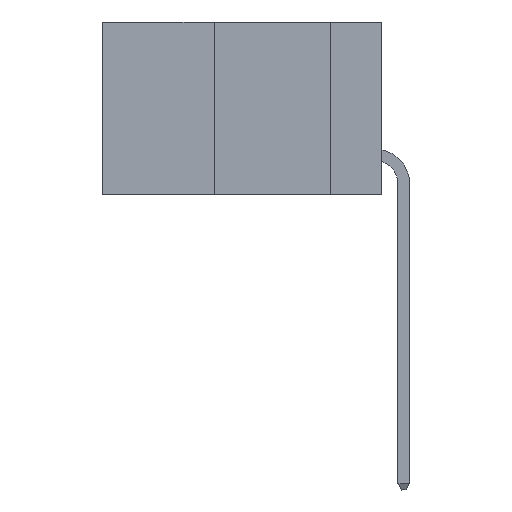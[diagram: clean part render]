
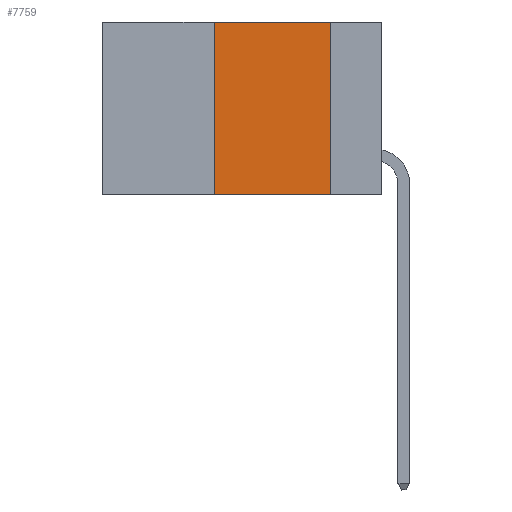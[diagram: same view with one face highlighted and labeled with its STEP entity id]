
A CAD part, left-side view. The second image highlights one B-rep face of the part: STEP entity #7759.
In plain terms, the highlighted planar face has unit normal (-1, 0, 0).
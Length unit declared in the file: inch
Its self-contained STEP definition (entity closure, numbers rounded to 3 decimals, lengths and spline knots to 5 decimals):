
#589 = EDGE_CURVE ( 'NONE', #13950, #16127, #8821, .T. ) ;
#635 = CARTESIAN_POINT ( 'NONE',  ( 0., 0.36, -0.37 ) ) ;
#652 = ORIENTED_EDGE ( 'NONE', *, *, #11546, .F. ) ;
#664 = CARTESIAN_POINT ( 'NONE',  ( 0., 0.6, -0.37 ) ) ;
#1356 = VECTOR ( 'NONE', #12120, 39.37008 ) ;
#2468 = VECTOR ( 'NONE', #7566, 39.37008 ) ;
#3319 = EDGE_CURVE ( 'NONE', #15656, #16127, #4731, .T. ) ;
#3501 = EDGE_LOOP ( 'NONE', ( #10491, #652, #5030, #10488 ) ) ;
#3700 = LINE ( 'NONE', #4114, #10033 ) ;
#3900 = CARTESIAN_POINT ( 'NONE',  ( 0., 0.6, 0. ) ) ;
#4114 = CARTESIAN_POINT ( 'NONE',  ( 0., 0.6, 0. ) ) ;
#4138 = CARTESIAN_POINT ( 'NONE',  ( 0., 0.36, 0. ) ) ;
#4293 = CARTESIAN_POINT ( 'NONE',  ( 0., 0.36, 0. ) ) ;
#4709 = VERTEX_POINT ( 'NONE', #4293 ) ;
#4731 = LINE ( 'NONE', #664, #1356 ) ;
#5030 = ORIENTED_EDGE ( 'NONE', *, *, #7220, .F. ) ;
#6456 = DIRECTION ( 'NONE',  ( 1., 0., 0. ) ) ;
#7220 = EDGE_CURVE ( 'NONE', #15656, #4709, #9380, .T. ) ;
#7566 = DIRECTION ( 'NONE',  ( 0., 0., -1. ) ) ;
#7759 = ADVANCED_FACE ( 'NONE', ( #15041 ), #11476, .F. ) ;
#8821 = LINE ( 'NONE', #15148, #2468 ) ;
#8979 = CARTESIAN_POINT ( 'NONE',  ( 0., 0.11, 0. ) ) ;
#8985 = DIRECTION ( 'NONE',  ( 0., 0., -1. ) ) ;
#9380 = LINE ( 'NONE', #4138, #12157 ) ;
#10033 = VECTOR ( 'NONE', #12933, 39.37008 ) ;
#10488 = ORIENTED_EDGE ( 'NONE', *, *, #3319, .T. ) ;
#10491 = ORIENTED_EDGE ( 'NONE', *, *, #589, .F. ) ;
#10588 = CARTESIAN_POINT ( 'NONE',  ( 0., 0.11, -0.37 ) ) ;
#11476 = PLANE ( 'NONE',  #13377 ) ;
#11546 = EDGE_CURVE ( 'NONE', #4709, #13950, #3700, .T. ) ;
#11601 = DIRECTION ( 'NONE',  ( 0., 0., 1. ) ) ;
#12120 = DIRECTION ( 'NONE',  ( 0., -1., 0. ) ) ;
#12157 = VECTOR ( 'NONE', #11601, 39.37008 ) ;
#12933 = DIRECTION ( 'NONE',  ( 0., -1., 0. ) ) ;
#13377 = AXIS2_PLACEMENT_3D ( 'NONE', #3900, #6456, #8985 ) ;
#13950 = VERTEX_POINT ( 'NONE', #8979 ) ;
#15041 = FACE_OUTER_BOUND ( 'NONE', #3501, .T. ) ;
#15148 = CARTESIAN_POINT ( 'NONE',  ( 0., 0.11, 0. ) ) ;
#15656 = VERTEX_POINT ( 'NONE', #635 ) ;
#16127 = VERTEX_POINT ( 'NONE', #10588 ) ;
